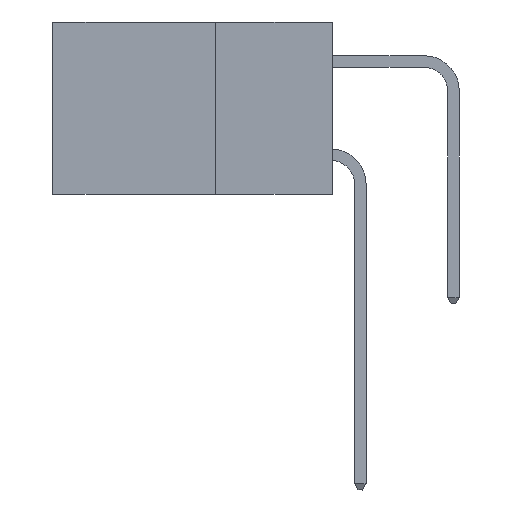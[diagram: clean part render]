
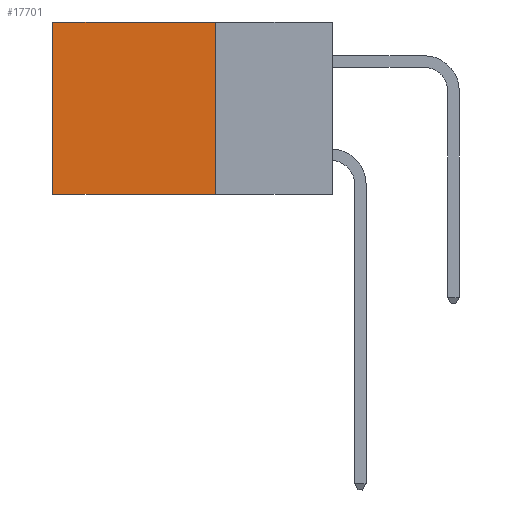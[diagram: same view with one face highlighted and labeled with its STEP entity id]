
A CAD part, left-side view. The second image highlights one B-rep face of the part: STEP entity #17701.
In plain terms, the highlighted planar face has unit normal (-1, 0, 0).
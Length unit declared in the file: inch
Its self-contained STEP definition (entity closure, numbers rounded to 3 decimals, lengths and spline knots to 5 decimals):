
#243 = VERTEX_POINT ( 'NONE', #12874 ) ;
#431 = EDGE_LOOP ( 'NONE', ( #7951, #16968, #17895, #7576 ) ) ;
#1248 = EDGE_CURVE ( 'NONE', #3582, #3111, #9384, .T. ) ;
#2018 = EDGE_CURVE ( 'NONE', #4434, #243, #6863, .T. ) ;
#2163 = VECTOR ( 'NONE', #6228, 39.37008 ) ;
#2954 = CARTESIAN_POINT ( 'NONE',  ( 0.298, 0.25, 0. ) ) ;
#3022 = VECTOR ( 'NONE', #11119, 39.37008 ) ;
#3111 = VERTEX_POINT ( 'NONE', #17518 ) ;
#3486 = FACE_OUTER_BOUND ( 'NONE', #431, .T. ) ;
#3582 = VERTEX_POINT ( 'NONE', #10346 ) ;
#3833 = CARTESIAN_POINT ( 'NONE',  ( 0.298, 0.6, 0. ) ) ;
#4434 = VERTEX_POINT ( 'NONE', #4695 ) ;
#4695 = CARTESIAN_POINT ( 'NONE',  ( 0.298, 0.6, 0. ) ) ;
#4855 = CARTESIAN_POINT ( 'NONE',  ( 0.298, 0.25, 0. ) ) ;
#5112 = DIRECTION ( 'NONE',  ( 0., 0., -1. ) ) ;
#6228 = DIRECTION ( 'NONE',  ( 0., 1., 0. ) ) ;
#6442 = EDGE_CURVE ( 'NONE', #3582, #4434, #10309, .T. ) ;
#6725 = DIRECTION ( 'NONE',  ( 0., 1., 0. ) ) ;
#6863 = LINE ( 'NONE', #3833, #3022 ) ;
#6977 = VECTOR ( 'NONE', #6725, 39.37008 ) ;
#7576 = ORIENTED_EDGE ( 'NONE', *, *, #6442, .T. ) ;
#7951 = ORIENTED_EDGE ( 'NONE', *, *, #2018, .T. ) ;
#9384 = LINE ( 'NONE', #4855, #11868 ) ;
#10309 = LINE ( 'NONE', #14647, #2163 ) ;
#10346 = CARTESIAN_POINT ( 'NONE',  ( 0.298, 0.25, 0. ) ) ;
#11119 = DIRECTION ( 'NONE',  ( 0., 0., -1. ) ) ;
#11802 = PLANE ( 'NONE',  #12997 ) ;
#11868 = VECTOR ( 'NONE', #5112, 39.37008 ) ;
#12874 = CARTESIAN_POINT ( 'NONE',  ( 0.298, 0.6, -0.37 ) ) ;
#12997 = AXIS2_PLACEMENT_3D ( 'NONE', #2954, #13069, #17438 ) ;
#13069 = DIRECTION ( 'NONE',  ( 1., 0., 0. ) ) ;
#13935 = CARTESIAN_POINT ( 'NONE',  ( 0.298, 0.25, -0.37 ) ) ;
#14319 = EDGE_CURVE ( 'NONE', #3111, #243, #16488, .T. ) ;
#14647 = CARTESIAN_POINT ( 'NONE',  ( 0.298, 0.25, 0. ) ) ;
#16488 = LINE ( 'NONE', #13935, #6977 ) ;
#16968 = ORIENTED_EDGE ( 'NONE', *, *, #14319, .F. ) ;
#17438 = DIRECTION ( 'NONE',  ( 0., 0., -1. ) ) ;
#17518 = CARTESIAN_POINT ( 'NONE',  ( 0.298, 0.25, -0.37 ) ) ;
#17701 = ADVANCED_FACE ( 'NONE', ( #3486 ), #11802, .F. ) ;
#17895 = ORIENTED_EDGE ( 'NONE', *, *, #1248, .F. ) ;
